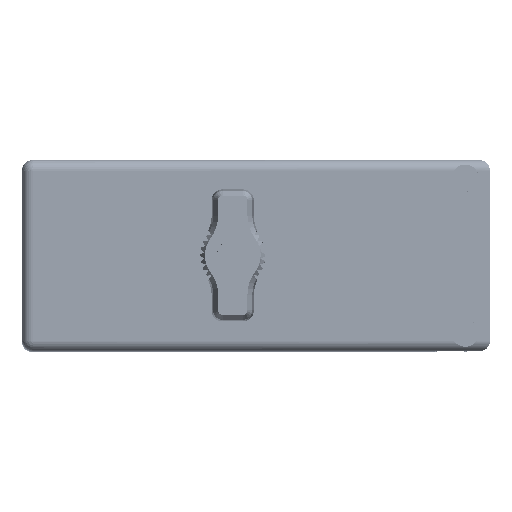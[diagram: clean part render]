
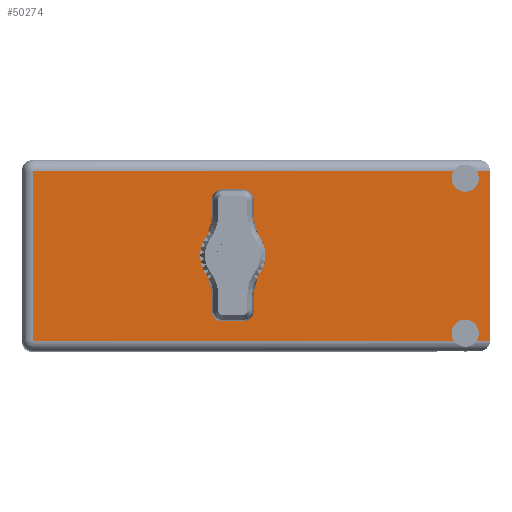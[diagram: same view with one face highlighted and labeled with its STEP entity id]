
A CAD part, top view. The second image highlights one B-rep face of the part: STEP entity #50274.
In plain terms, the highlighted face is planar.
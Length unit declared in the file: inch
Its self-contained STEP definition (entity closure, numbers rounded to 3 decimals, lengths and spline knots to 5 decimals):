
#802 = CARTESIAN_POINT ( 'NONE',  ( -1.359, 1.675, -0.547 ) ) ;
#1817 = EDGE_LOOP ( 'NONE', ( #34414, #43431 ) ) ;
#2247 = LINE ( 'NONE', #32611, #67641 ) ;
#2481 = EDGE_CURVE ( 'NONE', #33872, #13014, #4262, .T. ) ;
#3072 = CIRCLE ( 'NONE', #28561, 0.0875 ) ;
#4043 = ORIENTED_EDGE ( 'NONE', *, *, #37948, .F. ) ;
#4262 = LINE ( 'NONE', #82816, #51132 ) ;
#4814 = VECTOR ( 'NONE', #46653, 39.37008 ) ;
#5480 = EDGE_CURVE ( 'NONE', #73573, #15506, #19510, .T. ) ;
#5717 = EDGE_CURVE ( 'NONE', #22441, #13014, #2247, .T. ) ;
#7438 = FACE_BOUND ( 'NONE', #1817, .T. ) ;
#9253 = VERTEX_POINT ( 'NONE', #42335 ) ;
#9487 = AXIS2_PLACEMENT_3D ( 'NONE', #56478, #31350, #50886 ) ;
#9493 = DIRECTION ( 'NONE',  ( 0., 0., 1. ) ) ;
#10082 = CARTESIAN_POINT ( 'NONE',  ( 0., 1.675, 0.125 ) ) ;
#10965 = VERTEX_POINT ( 'NONE', #22077 ) ;
#12267 = EDGE_CURVE ( 'NONE', #9253, #73573, #49909, .T. ) ;
#13014 = VERTEX_POINT ( 'NONE', #29653 ) ;
#14893 = CARTESIAN_POINT ( 'NONE',  ( 1.499, 1.675, 0.5 ) ) ;
#15203 = CARTESIAN_POINT ( 'NONE',  ( 1.57281, 1.675, 0.547 ) ) ;
#15506 = VERTEX_POINT ( 'NONE', #28823 ) ;
#16373 = DIRECTION ( 'NONE',  ( -1., 0., 0. ) ) ;
#17373 = EDGE_CURVE ( 'NONE', #76655, #73831, #3072, .T. ) ;
#17429 = DIRECTION ( 'NONE',  ( 0., 1., 0. ) ) ;
#17524 = ORIENTED_EDGE ( 'NONE', *, *, #86675, .F. ) ;
#19510 = LINE ( 'NONE', #25957, #4814 ) ;
#20690 = AXIS2_PLACEMENT_3D ( 'NONE', #79599, #47092, #52613 ) ;
#22077 = CARTESIAN_POINT ( 'NONE',  ( 1.42519, 1.675, -0.547 ) ) ;
#22441 = VERTEX_POINT ( 'NONE', #15203 ) ;
#24203 = CARTESIAN_POINT ( 'NONE',  ( -1.289, 1.675, 0.547 ) ) ;
#24206 = CARTESIAN_POINT ( 'NONE',  ( 1.499, 1.675, -0.5 ) ) ;
#24797 = PLANE ( 'NONE',  #84287 ) ;
#25291 = CIRCLE ( 'NONE', #20690, 0.0875 ) ;
#25957 = CARTESIAN_POINT ( 'NONE',  ( 1.659, 1.675, 0.547 ) ) ;
#26652 = VECTOR ( 'NONE', #16373, 39.37008 ) ;
#28309 = CIRCLE ( 'NONE', #78147, 0.125 ) ;
#28561 = AXIS2_PLACEMENT_3D ( 'NONE', #24206, #82343, #48937 ) ;
#28823 = CARTESIAN_POINT ( 'NONE',  ( 1.42519, 1.675, 0.547 ) ) ;
#28947 = DIRECTION ( 'NONE',  ( 0., 0., 1. ) ) ;
#29653 = CARTESIAN_POINT ( 'NONE',  ( 1.659, 1.675, 0.547 ) ) ;
#30053 = DIRECTION ( 'NONE',  ( 0., 0., 1. ) ) ;
#30894 = CARTESIAN_POINT ( 'NONE',  ( -1.289, 1.675, -0.617 ) ) ;
#31350 = DIRECTION ( 'NONE',  ( 0., 1., 0. ) ) ;
#31870 = ORIENTED_EDGE ( 'NONE', *, *, #2481, .F. ) ;
#32606 = CARTESIAN_POINT ( 'NONE',  ( 1.499, 1.675, -0.4125 ) ) ;
#32611 = CARTESIAN_POINT ( 'NONE',  ( 1.659, 1.675, 0.547 ) ) ;
#33872 = VERTEX_POINT ( 'NONE', #85932 ) ;
#34414 = ORIENTED_EDGE ( 'NONE', *, *, #50606, .F. ) ;
#35952 = EDGE_CURVE ( 'NONE', #33872, #73831, #86242, .T. ) ;
#37948 = EDGE_CURVE ( 'NONE', #63894, #15506, #25291, .T. ) ;
#39357 = LINE ( 'NONE', #802, #82233 ) ;
#42234 = EDGE_CURVE ( 'NONE', #10965, #9253, #39357, .T. ) ;
#42335 = CARTESIAN_POINT ( 'NONE',  ( -1.289, 1.675, -0.547 ) ) ;
#42369 = CARTESIAN_POINT ( 'NONE',  ( -1.359, 1.675, -0.547 ) ) ;
#42463 = ORIENTED_EDGE ( 'NONE', *, *, #42234, .T. ) ;
#42658 = ORIENTED_EDGE ( 'NONE', *, *, #5480, .T. ) ;
#42846 = CARTESIAN_POINT ( 'NONE',  ( 0., 1.675, 0. ) ) ;
#43431 = ORIENTED_EDGE ( 'NONE', *, *, #67574, .F. ) ;
#43667 = VECTOR ( 'NONE', #77666, 39.37008 ) ;
#44103 = DIRECTION ( 'NONE',  ( 0., 1., 0. ) ) ;
#46653 = DIRECTION ( 'NONE',  ( 1., 0., 0. ) ) ;
#47092 = DIRECTION ( 'NONE',  ( 0., 1., 0. ) ) ;
#47193 = CARTESIAN_POINT ( 'NONE',  ( 1.57281, 1.675, -0.547 ) ) ;
#48413 = VERTEX_POINT ( 'NONE', #10082 ) ;
#48937 = DIRECTION ( 'NONE',  ( 0., 0., 1. ) ) ;
#49403 = CIRCLE ( 'NONE', #9487, 0.0875 ) ;
#49609 = ORIENTED_EDGE ( 'NONE', *, *, #65357, .F. ) ;
#49831 = CARTESIAN_POINT ( 'NONE',  ( 0., 1.675, 0. ) ) ;
#49909 = LINE ( 'NONE', #30894, #43667 ) ;
#50274 = ADVANCED_FACE ( 'NONE', ( #7438, #63918 ), #24797, .T. ) ;
#50606 = EDGE_CURVE ( 'NONE', #48413, #69319, #28309, .T. ) ;
#50886 = DIRECTION ( 'NONE',  ( 0., 0., 1. ) ) ;
#51132 = VECTOR ( 'NONE', #55851, 39.37008 ) ;
#51616 = ORIENTED_EDGE ( 'NONE', *, *, #5717, .T. ) ;
#52613 = DIRECTION ( 'NONE',  ( 0., 0., 1. ) ) ;
#55366 = CIRCLE ( 'NONE', #72414, 0.125 ) ;
#55851 = DIRECTION ( 'NONE',  ( 0., 0., 1. ) ) ;
#56478 = CARTESIAN_POINT ( 'NONE',  ( 1.499, 1.675, -0.5 ) ) ;
#58091 = CIRCLE ( 'NONE', #66979, 0.0875 ) ;
#60415 = DIRECTION ( 'NONE',  ( -1., 0., 0. ) ) ;
#62763 = CARTESIAN_POINT ( 'NONE',  ( 1.499, 1.675, 0.4125 ) ) ;
#63894 = VERTEX_POINT ( 'NONE', #62763 ) ;
#63918 = FACE_OUTER_BOUND ( 'NONE', #75413, .T. ) ;
#65357 = EDGE_CURVE ( 'NONE', #10965, #76655, #49403, .T. ) ;
#66979 = AXIS2_PLACEMENT_3D ( 'NONE', #14893, #83577, #28947 ) ;
#67574 = EDGE_CURVE ( 'NONE', #69319, #48413, #55366, .T. ) ;
#67641 = VECTOR ( 'NONE', #72684, 39.37008 ) ;
#69319 = VERTEX_POINT ( 'NONE', #79497 ) ;
#70661 = DIRECTION ( 'NONE',  ( 0., 1., 0. ) ) ;
#70712 = ORIENTED_EDGE ( 'NONE', *, *, #35952, .T. ) ;
#72414 = AXIS2_PLACEMENT_3D ( 'NONE', #49831, #70661, #30053 ) ;
#72684 = DIRECTION ( 'NONE',  ( 1., 0., 0. ) ) ;
#73573 = VERTEX_POINT ( 'NONE', #24203 ) ;
#73831 = VERTEX_POINT ( 'NONE', #47193 ) ;
#74074 = ORIENTED_EDGE ( 'NONE', *, *, #12267, .T. ) ;
#75413 = EDGE_LOOP ( 'NONE', ( #42658, #4043, #17524, #51616, #31870, #70712, #76904, #49609, #42463, #74074 ) ) ;
#76655 = VERTEX_POINT ( 'NONE', #32606 ) ;
#76904 = ORIENTED_EDGE ( 'NONE', *, *, #17373, .F. ) ;
#77450 = CARTESIAN_POINT ( 'NONE',  ( -1.359, 1.675, -0.617 ) ) ;
#77666 = DIRECTION ( 'NONE',  ( 0., 0., 1. ) ) ;
#78147 = AXIS2_PLACEMENT_3D ( 'NONE', #42846, #17429, #9493 ) ;
#79497 = CARTESIAN_POINT ( 'NONE',  ( 0., 1.675, -0.125 ) ) ;
#79599 = CARTESIAN_POINT ( 'NONE',  ( 1.499, 1.675, 0.5 ) ) ;
#82233 = VECTOR ( 'NONE', #60415, 39.37008 ) ;
#82343 = DIRECTION ( 'NONE',  ( 0., 1., 0. ) ) ;
#82816 = CARTESIAN_POINT ( 'NONE',  ( 1.659, 1.675, 0.617 ) ) ;
#83577 = DIRECTION ( 'NONE',  ( 0., 1., 0. ) ) ;
#84287 = AXIS2_PLACEMENT_3D ( 'NONE', #77450, #44103, #85272 ) ;
#85272 = DIRECTION ( 'NONE',  ( -1., 0., 0. ) ) ;
#85932 = CARTESIAN_POINT ( 'NONE',  ( 1.659, 1.675, -0.547 ) ) ;
#86242 = LINE ( 'NONE', #42369, #26652 ) ;
#86675 = EDGE_CURVE ( 'NONE', #22441, #63894, #58091, .T. ) ;
